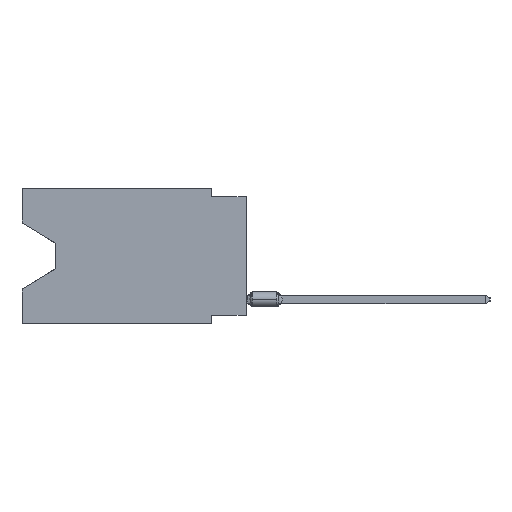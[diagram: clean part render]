
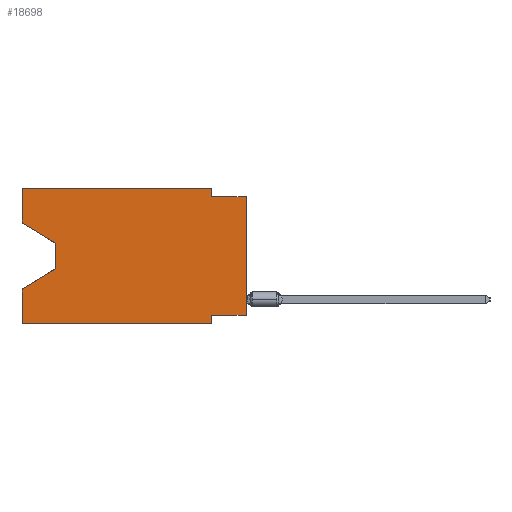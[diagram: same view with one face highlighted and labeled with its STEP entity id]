
A CAD part, left-side view. The second image highlights one B-rep face of the part: STEP entity #18698.
In plain terms, the highlighted planar face has unit normal (-1, 0, 0).
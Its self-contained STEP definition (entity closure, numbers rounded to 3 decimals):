
#550 = DIRECTION ( 'NONE',  ( 0., 0., -1. ) ) ;
#624 = VECTOR ( 'NONE', #23977, 1000. ) ;
#703 = LINE ( 'NONE', #4453, #13994 ) ;
#739 = EDGE_CURVE ( 'NONE', #18638, #35745, #13866, .T. ) ;
#1004 = VECTOR ( 'NONE', #13099, 1000. ) ;
#1038 = ORIENTED_EDGE ( 'NONE', *, *, #11059, .F. ) ;
#1965 = VERTEX_POINT ( 'NONE', #28895 ) ;
#2228 = EDGE_CURVE ( 'NONE', #3816, #38416, #12319, .T. ) ;
#2776 = EDGE_CURVE ( 'NONE', #35745, #29675, #36073, .T. ) ;
#2869 = CARTESIAN_POINT ( 'NONE',  ( 0., 13.97, -4.013 ) ) ;
#3455 = LINE ( 'NONE', #16266, #1004 ) ;
#3816 = VERTEX_POINT ( 'NONE', #18422 ) ;
#4078 = DIRECTION ( 'NONE',  ( 0., -0.855, -0.519 ) ) ;
#4453 = CARTESIAN_POINT ( 'NONE',  ( 0., 16.383, 0. ) ) ;
#4534 = CARTESIAN_POINT ( 'NONE',  ( 0., 0., -9.271 ) ) ;
#5107 = LINE ( 'NONE', #28007, #18544 ) ;
#5542 = LINE ( 'NONE', #21899, #21773 ) ;
#6954 = EDGE_CURVE ( 'NONE', #26192, #29675, #5542, .T. ) ;
#7703 = DIRECTION ( 'NONE',  ( 1., 0., 0. ) ) ;
#8115 = ORIENTED_EDGE ( 'NONE', *, *, #739, .F. ) ;
#8728 = CARTESIAN_POINT ( 'NONE',  ( 0., 16.383, 0. ) ) ;
#9087 = VERTEX_POINT ( 'NONE', #23109 ) ;
#9657 = ORIENTED_EDGE ( 'NONE', *, *, #2228, .T. ) ;
#9754 = ORIENTED_EDGE ( 'NONE', *, *, #33661, .T. ) ;
#10304 = EDGE_CURVE ( 'NONE', #18638, #1965, #23087, .T. ) ;
#10356 = DIRECTION ( 'NONE',  ( 0., 0., 1. ) ) ;
#11059 = EDGE_CURVE ( 'NONE', #20702, #30311, #13693, .T. ) ;
#11819 = DIRECTION ( 'NONE',  ( 0., -1., 0. ) ) ;
#12062 = LINE ( 'NONE', #8728, #21308 ) ;
#12186 = AXIS2_PLACEMENT_3D ( 'NONE', #36501, #7703, #31426 ) ;
#12319 = LINE ( 'NONE', #2869, #26295 ) ;
#13099 = DIRECTION ( 'NONE',  ( 0., -1., 0. ) ) ;
#13557 = CARTESIAN_POINT ( 'NONE',  ( 0., 2.54, -9.906 ) ) ;
#13693 = LINE ( 'NONE', #17052, #624 ) ;
#13866 = LINE ( 'NONE', #16822, #20407 ) ;
#13994 = VECTOR ( 'NONE', #10356, 1000. ) ;
#14525 = EDGE_CURVE ( 'NONE', #26192, #22302, #12062, .T. ) ;
#16266 = CARTESIAN_POINT ( 'NONE',  ( 0., 0., -0.635 ) ) ;
#16295 = CARTESIAN_POINT ( 'NONE',  ( 0., 16.383, -9.906 ) ) ;
#16822 = CARTESIAN_POINT ( 'NONE',  ( 0., 0., -9.271 ) ) ;
#17052 = CARTESIAN_POINT ( 'NONE',  ( 0., 2.54, 0. ) ) ;
#18422 = CARTESIAN_POINT ( 'NONE',  ( 0., 13.97, -4.013 ) ) ;
#18544 = VECTOR ( 'NONE', #11819, 1000. ) ;
#18638 = VERTEX_POINT ( 'NONE', #4534 ) ;
#18698 = ADVANCED_FACE ( 'NONE', ( #33129 ), #26824, .F. ) ;
#19675 = EDGE_CURVE ( 'NONE', #40815, #20702, #5107, .T. ) ;
#20407 = VECTOR ( 'NONE', #22713, 1000. ) ;
#20635 = ORIENTED_EDGE ( 'NONE', *, *, #23571, .T. ) ;
#20702 = VERTEX_POINT ( 'NONE', #39242 ) ;
#20987 = ORIENTED_EDGE ( 'NONE', *, *, #2776, .F. ) ;
#21097 = EDGE_LOOP ( 'NONE', ( #9754, #9657, #20635, #32718, #28624, #20987, #8115, #24514, #31790, #1038, #25552, #32500 ) ) ;
#21308 = VECTOR ( 'NONE', #41286, 1000. ) ;
#21773 = VECTOR ( 'NONE', #40655, 1000. ) ;
#21899 = CARTESIAN_POINT ( 'NONE',  ( 0., 16.383, -9.906 ) ) ;
#22119 = VECTOR ( 'NONE', #550, 1000. ) ;
#22302 = VERTEX_POINT ( 'NONE', #31293 ) ;
#22713 = DIRECTION ( 'NONE',  ( 0., 1., 0. ) ) ;
#23087 = LINE ( 'NONE', #32777, #36202 ) ;
#23109 = CARTESIAN_POINT ( 'NONE',  ( 0., 16.383, -2.546 ) ) ;
#23121 = CARTESIAN_POINT ( 'NONE',  ( 0., 13.97, -5.893 ) ) ;
#23571 = EDGE_CURVE ( 'NONE', #38416, #22302, #25349, .T. ) ;
#23977 = DIRECTION ( 'NONE',  ( 0., 0., -1. ) ) ;
#24514 = ORIENTED_EDGE ( 'NONE', *, *, #10304, .T. ) ;
#25349 = LINE ( 'NONE', #38222, #36148 ) ;
#25552 = ORIENTED_EDGE ( 'NONE', *, *, #19675, .F. ) ;
#26192 = VERTEX_POINT ( 'NONE', #16295 ) ;
#26295 = VECTOR ( 'NONE', #31033, 1000. ) ;
#26824 = PLANE ( 'NONE',  #12186 ) ;
#26965 = LINE ( 'NONE', #29503, #34635 ) ;
#28007 = CARTESIAN_POINT ( 'NONE',  ( 0., 16.383, 0. ) ) ;
#28526 = EDGE_CURVE ( 'NONE', #30311, #1965, #3455, .T. ) ;
#28624 = ORIENTED_EDGE ( 'NONE', *, *, #6954, .T. ) ;
#28895 = CARTESIAN_POINT ( 'NONE',  ( 0., 0., -0.635 ) ) ;
#29503 = CARTESIAN_POINT ( 'NONE',  ( 0., 16.383, -2.546 ) ) ;
#29675 = VERTEX_POINT ( 'NONE', #35193 ) ;
#30311 = VERTEX_POINT ( 'NONE', #30607 ) ;
#30607 = CARTESIAN_POINT ( 'NONE',  ( 0., 2.54, -0.635 ) ) ;
#31033 = DIRECTION ( 'NONE',  ( 0., 0., -1. ) ) ;
#31293 = CARTESIAN_POINT ( 'NONE',  ( 0., 16.383, -7.36 ) ) ;
#31426 = DIRECTION ( 'NONE',  ( 0., 0., -1. ) ) ;
#31790 = ORIENTED_EDGE ( 'NONE', *, *, #28526, .F. ) ;
#32035 = EDGE_CURVE ( 'NONE', #9087, #40815, #703, .T. ) ;
#32500 = ORIENTED_EDGE ( 'NONE', *, *, #32035, .F. ) ;
#32718 = ORIENTED_EDGE ( 'NONE', *, *, #14525, .F. ) ;
#32777 = CARTESIAN_POINT ( 'NONE',  ( 0., 0., 0. ) ) ;
#33129 = FACE_OUTER_BOUND ( 'NONE', #21097, .T. ) ;
#33191 = DIRECTION ( 'NONE',  ( 0., 0., 1. ) ) ;
#33661 = EDGE_CURVE ( 'NONE', #9087, #3816, #26965, .T. ) ;
#34158 = CARTESIAN_POINT ( 'NONE',  ( 0., 16.383, 0. ) ) ;
#34635 = VECTOR ( 'NONE', #4078, 1000. ) ;
#34852 = DIRECTION ( 'NONE',  ( 0., 0.855, -0.519 ) ) ;
#35193 = CARTESIAN_POINT ( 'NONE',  ( 0., 2.54, -9.906 ) ) ;
#35745 = VERTEX_POINT ( 'NONE', #38656 ) ;
#36073 = LINE ( 'NONE', #13557, #22119 ) ;
#36148 = VECTOR ( 'NONE', #34852, 1000. ) ;
#36202 = VECTOR ( 'NONE', #33191, 1000. ) ;
#36501 = CARTESIAN_POINT ( 'NONE',  ( 0., 16.383, 0. ) ) ;
#38222 = CARTESIAN_POINT ( 'NONE',  ( 0., 13.97, -5.893 ) ) ;
#38416 = VERTEX_POINT ( 'NONE', #23121 ) ;
#38656 = CARTESIAN_POINT ( 'NONE',  ( 0., 2.54, -9.271 ) ) ;
#39242 = CARTESIAN_POINT ( 'NONE',  ( 0., 2.54, 0. ) ) ;
#40655 = DIRECTION ( 'NONE',  ( 0., -1., 0. ) ) ;
#40815 = VERTEX_POINT ( 'NONE', #34158 ) ;
#41286 = DIRECTION ( 'NONE',  ( 0., 0., 1. ) ) ;
